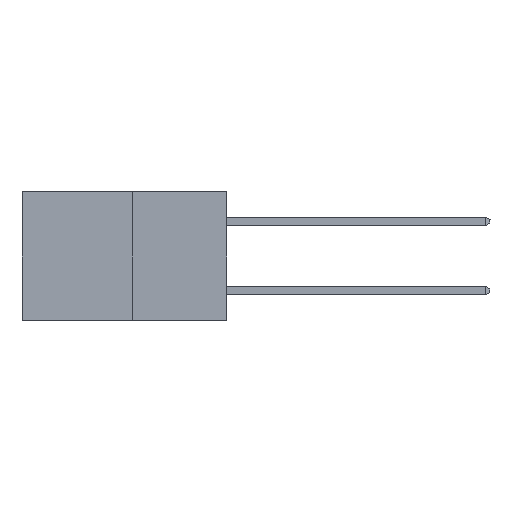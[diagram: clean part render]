
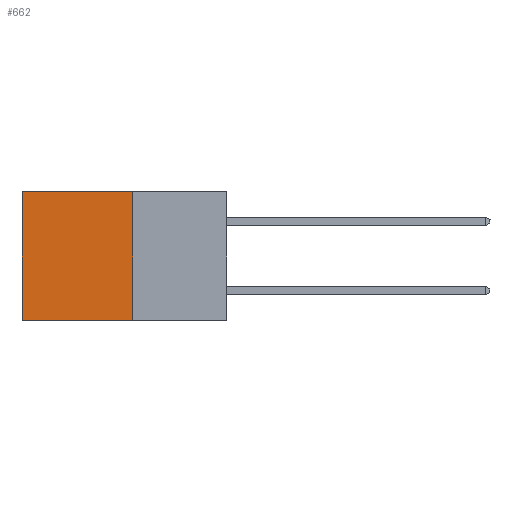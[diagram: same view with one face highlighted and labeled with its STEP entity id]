
A CAD part, left-side view. The second image highlights one B-rep face of the part: STEP entity #662.
In plain terms, the highlighted planar face has unit normal (-1, 0, 0).
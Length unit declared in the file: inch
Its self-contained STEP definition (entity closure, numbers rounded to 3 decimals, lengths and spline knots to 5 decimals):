
#136 = CARTESIAN_POINT ( 'NONE',  ( 0.277, 0.59, -0.37 ) ) ;
#590 = CARTESIAN_POINT ( 'NONE',  ( 0.277, 0.27, -0.37 ) ) ;
#662 = ADVANCED_FACE ( 'NONE', ( #19522 ), #5544, .F. ) ;
#1064 = LINE ( 'NONE', #18476, #9049 ) ;
#1116 = VERTEX_POINT ( 'NONE', #2738 ) ;
#1970 = ORIENTED_EDGE ( 'NONE', *, *, #19279, .T. ) ;
#2096 = VERTEX_POINT ( 'NONE', #590 ) ;
#2339 = ORIENTED_EDGE ( 'NONE', *, *, #17415, .F. ) ;
#2738 = CARTESIAN_POINT ( 'NONE',  ( 0.277, 0.59, 0. ) ) ;
#3777 = EDGE_LOOP ( 'NONE', ( #11864, #2339, #10794, #1970 ) ) ;
#3891 = CARTESIAN_POINT ( 'NONE',  ( 0.277, 0.27, -0.37 ) ) ;
#3964 = VERTEX_POINT ( 'NONE', #136 ) ;
#5354 = VECTOR ( 'NONE', #18390, 39.37008 ) ;
#5393 = VERTEX_POINT ( 'NONE', #12122 ) ;
#5544 = PLANE ( 'NONE',  #12152 ) ;
#5666 = DIRECTION ( 'NONE',  ( 0., 1., 0. ) ) ;
#5795 = CARTESIAN_POINT ( 'NONE',  ( 0.277, 0.27, 0. ) ) ;
#7570 = CARTESIAN_POINT ( 'NONE',  ( 0.277, 0.59, -0.37 ) ) ;
#9049 = VECTOR ( 'NONE', #18926, 39.37008 ) ;
#9053 = DIRECTION ( 'NONE',  ( 0., 1., 0. ) ) ;
#9170 = CARTESIAN_POINT ( 'NONE',  ( 0.277, 0.27, -0.37 ) ) ;
#9736 = VECTOR ( 'NONE', #9053, 39.37008 ) ;
#10794 = ORIENTED_EDGE ( 'NONE', *, *, #14292, .F. ) ;
#11864 = ORIENTED_EDGE ( 'NONE', *, *, #12766, .T. ) ;
#11937 = LINE ( 'NONE', #5795, #19939 ) ;
#12122 = CARTESIAN_POINT ( 'NONE',  ( 0.277, 0.27, 0. ) ) ;
#12152 = AXIS2_PLACEMENT_3D ( 'NONE', #3891, #18149, #17530 ) ;
#12766 = EDGE_CURVE ( 'NONE', #1116, #3964, #18133, .T. ) ;
#13564 = LINE ( 'NONE', #9170, #9736 ) ;
#14292 = EDGE_CURVE ( 'NONE', #5393, #2096, #1064, .T. ) ;
#17415 = EDGE_CURVE ( 'NONE', #2096, #3964, #13564, .T. ) ;
#17530 = DIRECTION ( 'NONE',  ( 0., 0., -1. ) ) ;
#18133 = LINE ( 'NONE', #7570, #5354 ) ;
#18149 = DIRECTION ( 'NONE',  ( 1., 0., 0. ) ) ;
#18390 = DIRECTION ( 'NONE',  ( 0., 0., -1. ) ) ;
#18476 = CARTESIAN_POINT ( 'NONE',  ( 0.277, 0.27, -0.37 ) ) ;
#18926 = DIRECTION ( 'NONE',  ( 0., 0., -1. ) ) ;
#19279 = EDGE_CURVE ( 'NONE', #5393, #1116, #11937, .T. ) ;
#19522 = FACE_OUTER_BOUND ( 'NONE', #3777, .T. ) ;
#19939 = VECTOR ( 'NONE', #5666, 39.37008 ) ;
